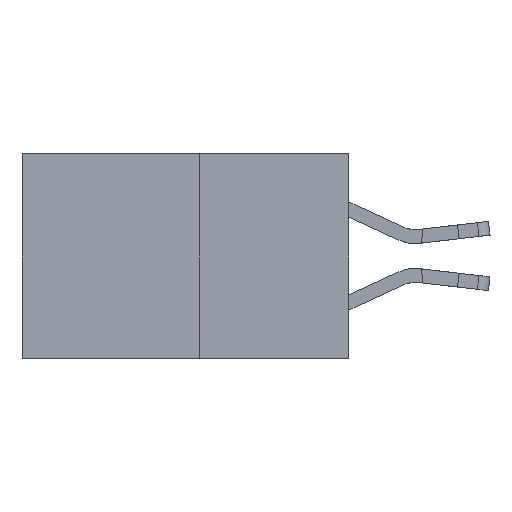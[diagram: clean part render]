
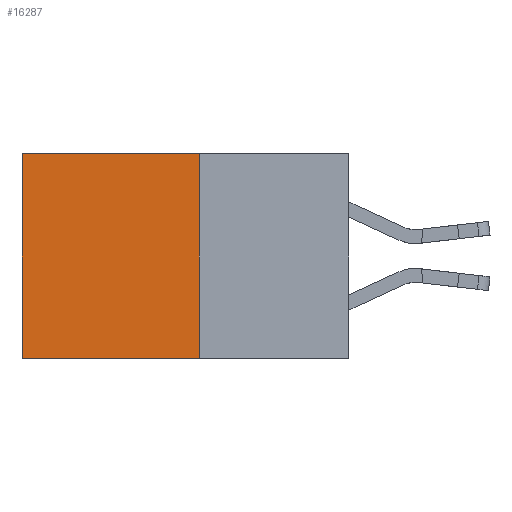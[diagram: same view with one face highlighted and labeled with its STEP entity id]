
A CAD part, left-side view. The second image highlights one B-rep face of the part: STEP entity #16287.
In plain terms, the highlighted planar face has unit normal (-1, 0, 0).
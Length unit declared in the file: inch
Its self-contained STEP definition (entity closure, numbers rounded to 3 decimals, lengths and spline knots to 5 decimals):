
#506 = VECTOR ( 'NONE', #13010, 39.37008 ) ;
#648 = LINE ( 'NONE', #949, #7273 ) ;
#924 = DIRECTION ( 'NONE',  ( 0., 0., -1. ) ) ;
#949 = CARTESIAN_POINT ( 'NONE',  ( 0.277, 0.59, -0.37 ) ) ;
#2013 = ORIENTED_EDGE ( 'NONE', *, *, #15633, .F. ) ;
#2502 = VECTOR ( 'NONE', #5513, 39.37008 ) ;
#2567 = EDGE_CURVE ( 'NONE', #13049, #16158, #648, .T. ) ;
#2828 = CARTESIAN_POINT ( 'NONE',  ( 0.277, 0.27, -0.37 ) ) ;
#4160 = CARTESIAN_POINT ( 'NONE',  ( 0.277, 0.27, -0.37 ) ) ;
#4526 = LINE ( 'NONE', #2828, #506 ) ;
#5460 = CARTESIAN_POINT ( 'NONE',  ( 0.277, 0.27, -0.37 ) ) ;
#5475 = DIRECTION ( 'NONE',  ( 0., 0., -1. ) ) ;
#5513 = DIRECTION ( 'NONE',  ( 0., 1., 0. ) ) ;
#5667 = CARTESIAN_POINT ( 'NONE',  ( 0.277, 0.27, -0.37 ) ) ;
#6269 = CARTESIAN_POINT ( 'NONE',  ( 0.277, 0.27, 0. ) ) ;
#7273 = VECTOR ( 'NONE', #924, 39.37008 ) ;
#7957 = VECTOR ( 'NONE', #10623, 39.37008 ) ;
#8564 = ORIENTED_EDGE ( 'NONE', *, *, #14244, .F. ) ;
#9264 = PLANE ( 'NONE',  #14813 ) ;
#9918 = VERTEX_POINT ( 'NONE', #6269 ) ;
#10239 = EDGE_CURVE ( 'NONE', #9918, #13049, #14887, .T. ) ;
#10623 = DIRECTION ( 'NONE',  ( 0., 1., 0. ) ) ;
#10667 = FACE_OUTER_BOUND ( 'NONE', #15178, .T. ) ;
#10675 = CARTESIAN_POINT ( 'NONE',  ( 0.277, 0.27, 0. ) ) ;
#11571 = CARTESIAN_POINT ( 'NONE',  ( 0.277, 0.59, -0.37 ) ) ;
#11691 = VERTEX_POINT ( 'NONE', #5667 ) ;
#12290 = ORIENTED_EDGE ( 'NONE', *, *, #10239, .T. ) ;
#12686 = LINE ( 'NONE', #5460, #2502 ) ;
#12992 = DIRECTION ( 'NONE',  ( 1., 0., 0. ) ) ;
#13010 = DIRECTION ( 'NONE',  ( 0., 0., -1. ) ) ;
#13049 = VERTEX_POINT ( 'NONE', #13221 ) ;
#13221 = CARTESIAN_POINT ( 'NONE',  ( 0.277, 0.59, 0. ) ) ;
#14244 = EDGE_CURVE ( 'NONE', #11691, #16158, #12686, .T. ) ;
#14710 = ORIENTED_EDGE ( 'NONE', *, *, #2567, .T. ) ;
#14813 = AXIS2_PLACEMENT_3D ( 'NONE', #4160, #12992, #5475 ) ;
#14887 = LINE ( 'NONE', #10675, #7957 ) ;
#15178 = EDGE_LOOP ( 'NONE', ( #14710, #8564, #2013, #12290 ) ) ;
#15633 = EDGE_CURVE ( 'NONE', #9918, #11691, #4526, .T. ) ;
#16158 = VERTEX_POINT ( 'NONE', #11571 ) ;
#16287 = ADVANCED_FACE ( 'NONE', ( #10667 ), #9264, .F. ) ;
